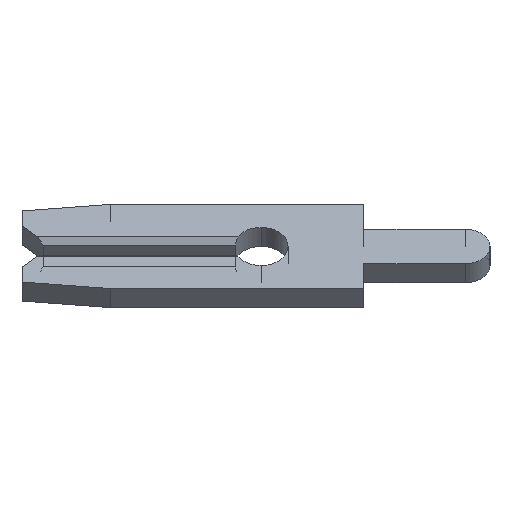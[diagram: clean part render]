
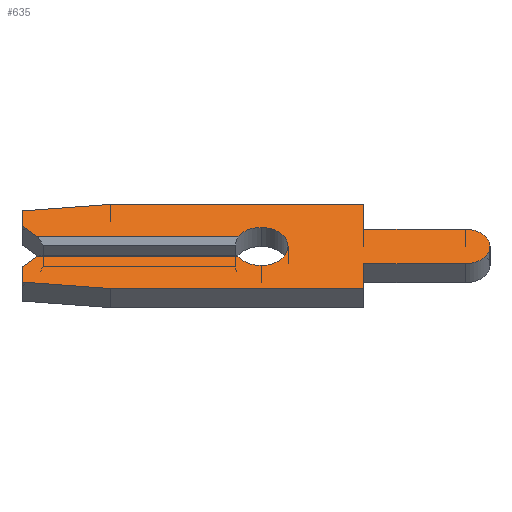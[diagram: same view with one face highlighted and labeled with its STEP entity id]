
A CAD part, left-side view. The second image highlights one B-rep face of the part: STEP entity #635.
In plain terms, the highlighted face is planar.
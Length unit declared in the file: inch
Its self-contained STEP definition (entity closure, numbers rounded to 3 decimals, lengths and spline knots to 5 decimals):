
#38 = EDGE_CURVE ( 'NONE', #1120, #1003, #626, .T. ) ;
#79 = EDGE_CURVE ( 'NONE', #2092, #1792, #140, .T. ) ;
#87 = VERTEX_POINT ( 'NONE', #257 ) ;
#112 = VECTOR ( 'NONE', #1961, 39.37008 ) ;
#115 = VERTEX_POINT ( 'NONE', #1162 ) ;
#116 = CARTESIAN_POINT ( 'NONE',  ( -0.013, -0.099, -0.0575 ) ) ;
#125 = CARTESIAN_POINT ( 'NONE',  ( -0.013, 0.231, 0.04857 ) ) ;
#134 = DIRECTION ( 'NONE',  ( 0., -1., 0. ) ) ;
#140 = CIRCLE ( 'NONE', #2225, 0.026 ) ;
#150 = VERTEX_POINT ( 'NONE', #699 ) ;
#176 = CARTESIAN_POINT ( 'NONE',  ( -0.013, 0.146, -0.0575 ) ) ;
#189 = ORIENTED_EDGE ( 'NONE', *, *, #464, .F. ) ;
#194 = VERTEX_POINT ( 'NONE', #485 ) ;
#195 = EDGE_CURVE ( 'NONE', #227, #2071, #1377, .T. ) ;
#225 = VECTOR ( 'NONE', #446, 39.37008 ) ;
#227 = VERTEX_POINT ( 'NONE', #308 ) ;
#232 = ORIENTED_EDGE ( 'NONE', *, *, #1086, .F. ) ;
#257 = CARTESIAN_POINT ( 'NONE',  ( -0.013, 0.231, 0.028 ) ) ;
#308 = CARTESIAN_POINT ( 'NONE',  ( -0.013, 0.231, 0.04857 ) ) ;
#312 = VECTOR ( 'NONE', #756, 39.37008 ) ;
#326 = EDGE_CURVE ( 'NONE', #115, #2092, #964, .T. ) ;
#348 = DIRECTION ( 'NONE',  ( 0., 0.707, 0.707 ) ) ;
#369 = DIRECTION ( 'NONE',  ( 0., 0.995, 0.105 ) ) ;
#387 = CARTESIAN_POINT ( 'NONE',  ( -0.013, -0.099, -0.0235 ) ) ;
#400 = CARTESIAN_POINT ( 'NONE',  ( -0.013, -0.1975, -0.0235 ) ) ;
#416 = DIRECTION ( 'NONE',  ( 0., 0., 1. ) ) ;
#424 = VECTOR ( 'NONE', #671, 39.37008 ) ;
#426 = CARTESIAN_POINT ( 'NONE',  ( -0.013, 0., 0. ) ) ;
#443 = CARTESIAN_POINT ( 'NONE',  ( -0.013, -0.099, -0.0235 ) ) ;
#446 = DIRECTION ( 'NONE',  ( 0., -1., 0. ) ) ;
#450 = EDGE_CURVE ( 'NONE', #1792, #150, #1846, .T. ) ;
#464 = EDGE_CURVE ( 'NONE', #150, #2282, #1625, .T. ) ;
#485 = CARTESIAN_POINT ( 'NONE',  ( -0.013, -0.099, 0.0575 ) ) ;
#487 = ORIENTED_EDGE ( 'NONE', *, *, #1054, .F. ) ;
#493 = EDGE_CURVE ( 'NONE', #87, #227, #1459, .T. ) ;
#513 = VECTOR ( 'NONE', #134, 39.37008 ) ;
#520 = ORIENTED_EDGE ( 'NONE', *, *, #450, .F. ) ;
#523 = DIRECTION ( 'NONE',  ( -1., 0., 0. ) ) ;
#560 = AXIS2_PLACEMENT_3D ( 'NONE', #2026, #946, #416 ) ;
#565 = LINE ( 'NONE', #848, #1104 ) ;
#591 = LINE ( 'NONE', #1221, #1989 ) ;
#601 = VERTEX_POINT ( 'NONE', #2160 ) ;
#602 = EDGE_CURVE ( 'NONE', #1603, #87, #1551, .T. ) ;
#626 = LINE ( 'NONE', #1579, #225 ) ;
#634 = DIRECTION ( 'NONE',  ( 0., -0.707, 0.707 ) ) ;
#635 = ADVANCED_FACE ( 'NONE', ( #906 ), #730, .F. ) ;
#647 = EDGE_CURVE ( 'NONE', #1382, #921, #1400, .T. ) ;
#671 = DIRECTION ( 'NONE',  ( 0., -0.995, 0.105 ) ) ;
#684 = DIRECTION ( 'NONE',  ( 0., 0., -1. ) ) ;
#686 = ORIENTED_EDGE ( 'NONE', *, *, #326, .F. ) ;
#690 = ORIENTED_EDGE ( 'NONE', *, *, #701, .F. ) ;
#699 = CARTESIAN_POINT ( 'NONE',  ( -0.013, 0., 0.026 ) ) ;
#701 = EDGE_CURVE ( 'NONE', #921, #601, #2284, .T. ) ;
#705 = VECTOR ( 'NONE', #634, 39.37008 ) ;
#729 = LINE ( 'NONE', #116, #1910 ) ;
#730 = PLANE ( 'NONE',  #1295 ) ;
#734 = ORIENTED_EDGE ( 'NONE', *, *, #1749, .F. ) ;
#738 = ORIENTED_EDGE ( 'NONE', *, *, #2148, .F. ) ;
#756 = DIRECTION ( 'NONE',  ( 0., 0., 1. ) ) ;
#786 = LINE ( 'NONE', #1552, #705 ) ;
#816 = ORIENTED_EDGE ( 'NONE', *, *, #647, .F. ) ;
#848 = CARTESIAN_POINT ( 'NONE',  ( -0.013, -0.099, 0.0575 ) ) ;
#876 = DIRECTION ( 'NONE',  ( 0., -1., 0. ) ) ;
#879 = ORIENTED_EDGE ( 'NONE', *, *, #493, .F. ) ;
#880 = VECTOR ( 'NONE', #348, 39.37008 ) ;
#893 = DIRECTION ( 'NONE',  ( 0., 1., 0. ) ) ;
#906 = FACE_OUTER_BOUND ( 'NONE', #2083, .T. ) ;
#907 = CARTESIAN_POINT ( 'NONE',  ( -0.013, 0., 0. ) ) ;
#921 = VERTEX_POINT ( 'NONE', #2195 ) ;
#936 = CARTESIAN_POINT ( 'NONE',  ( -0.013, 0.231, -0.028 ) ) ;
#946 = DIRECTION ( 'NONE',  ( 1., 0., 0. ) ) ;
#963 = CARTESIAN_POINT ( 'NONE',  ( -0.013, -0.099, -0.0575 ) ) ;
#964 = LINE ( 'NONE', #1526, #513 ) ;
#998 = VECTOR ( 'NONE', #369, 39.37008 ) ;
#1001 = AXIS2_PLACEMENT_3D ( 'NONE', #1237, #523, #1784 ) ;
#1003 = VERTEX_POINT ( 'NONE', #2171 ) ;
#1017 = EDGE_CURVE ( 'NONE', #1003, #1312, #2193, .T. ) ;
#1032 = DIRECTION ( 'NONE',  ( 0., 0., -1. ) ) ;
#1039 = CARTESIAN_POINT ( 'NONE',  ( -0.013, 0.231, 0.013 ) ) ;
#1046 = AXIS2_PLACEMENT_3D ( 'NONE', #2166, #1954, #684 ) ;
#1051 = CARTESIAN_POINT ( 'NONE',  ( -0.013, 0.231, 0.028 ) ) ;
#1052 = ORIENTED_EDGE ( 'NONE', *, *, #2218, .F. ) ;
#1054 = EDGE_CURVE ( 'NONE', #1312, #1431, #2306, .T. ) ;
#1086 = EDGE_CURVE ( 'NONE', #601, #1203, #1816, .T. ) ;
#1104 = VECTOR ( 'NONE', #2132, 39.37008 ) ;
#1120 = VERTEX_POINT ( 'NONE', #1131 ) ;
#1131 = CARTESIAN_POINT ( 'NONE',  ( -0.013, -0.099, 0.0235 ) ) ;
#1162 = CARTESIAN_POINT ( 'NONE',  ( -0.013, 0.216, -0.013 ) ) ;
#1177 = ORIENTED_EDGE ( 'NONE', *, *, #1017, .F. ) ;
#1183 = ORIENTED_EDGE ( 'NONE', *, *, #195, .F. ) ;
#1203 = VERTEX_POINT ( 'NONE', #2032 ) ;
#1221 = CARTESIAN_POINT ( 'NONE',  ( -0.013, 0.146, 0.0575 ) ) ;
#1225 = DIRECTION ( 'NONE',  ( 0., -1., 0. ) ) ;
#1234 = CARTESIAN_POINT ( 'NONE',  ( -0.013, 0.02252, -0.013 ) ) ;
#1237 = CARTESIAN_POINT ( 'NONE',  ( -0.013, 0., 0. ) ) ;
#1264 = ORIENTED_EDGE ( 'NONE', *, *, #38, .F. ) ;
#1267 = CARTESIAN_POINT ( 'NONE',  ( -0.013, 0.02252, 0.013 ) ) ;
#1295 = AXIS2_PLACEMENT_3D ( 'NONE', #907, #2002, #2182 ) ;
#1312 = VERTEX_POINT ( 'NONE', #400 ) ;
#1324 = ORIENTED_EDGE ( 'NONE', *, *, #602, .F. ) ;
#1359 = DIRECTION ( 'NONE',  ( -1., 0., 0. ) ) ;
#1377 = LINE ( 'NONE', #125, #424 ) ;
#1382 = VERTEX_POINT ( 'NONE', #963 ) ;
#1400 = LINE ( 'NONE', #176, #2227 ) ;
#1431 = VERTEX_POINT ( 'NONE', #443 ) ;
#1459 = LINE ( 'NONE', #1051, #112 ) ;
#1471 = CARTESIAN_POINT ( 'NONE',  ( -0.013, 0.231, -0.04857 ) ) ;
#1515 = VECTOR ( 'NONE', #1225, 39.37008 ) ;
#1517 = ORIENTED_EDGE ( 'NONE', *, *, #2161, .T. ) ;
#1526 = CARTESIAN_POINT ( 'NONE',  ( -0.013, 0., -0.013 ) ) ;
#1547 = LINE ( 'NONE', #1039, #1515 ) ;
#1551 = LINE ( 'NONE', #1588, #880 ) ;
#1552 = CARTESIAN_POINT ( 'NONE',  ( -0.013, 0.2105, -0.0075 ) ) ;
#1579 = CARTESIAN_POINT ( 'NONE',  ( -0.013, -0.099, 0.0235 ) ) ;
#1588 = CARTESIAN_POINT ( 'NONE',  ( -0.013, 0.2105, 0.0075 ) ) ;
#1603 = VERTEX_POINT ( 'NONE', #1720 ) ;
#1625 = CIRCLE ( 'NONE', #1001, 0.026 ) ;
#1720 = CARTESIAN_POINT ( 'NONE',  ( -0.013, 0.216, 0.013 ) ) ;
#1741 = VECTOR ( 'NONE', #893, 39.37008 ) ;
#1749 = EDGE_CURVE ( 'NONE', #1203, #115, #786, .T. ) ;
#1750 = CARTESIAN_POINT ( 'NONE',  ( -0.013, 0.146, 0.0575 ) ) ;
#1784 = DIRECTION ( 'NONE',  ( 0., 0., -1. ) ) ;
#1792 = VERTEX_POINT ( 'NONE', #1911 ) ;
#1808 = DIRECTION ( 'NONE',  ( 0., 1., 0. ) ) ;
#1816 = LINE ( 'NONE', #936, #312 ) ;
#1846 = CIRCLE ( 'NONE', #1046, 0.026 ) ;
#1875 = ORIENTED_EDGE ( 'NONE', *, *, #2035, .F. ) ;
#1910 = VECTOR ( 'NONE', #2116, 39.37008 ) ;
#1911 = CARTESIAN_POINT ( 'NONE',  ( -0.013, 0., -0.026 ) ) ;
#1920 = ORIENTED_EDGE ( 'NONE', *, *, #79, .F. ) ;
#1954 = DIRECTION ( 'NONE',  ( -1., 0., 0. ) ) ;
#1961 = DIRECTION ( 'NONE',  ( 0., 0., 1. ) ) ;
#1989 = VECTOR ( 'NONE', #876, 39.37008 ) ;
#2002 = DIRECTION ( 'NONE',  ( 1., 0., 0. ) ) ;
#2026 = CARTESIAN_POINT ( 'NONE',  ( -0.013, -0.1975, 0. ) ) ;
#2032 = CARTESIAN_POINT ( 'NONE',  ( -0.013, 0.231, -0.028 ) ) ;
#2035 = EDGE_CURVE ( 'NONE', #1431, #1382, #729, .T. ) ;
#2071 = VERTEX_POINT ( 'NONE', #1750 ) ;
#2083 = EDGE_LOOP ( 'NONE', ( #1517, #189, #520, #1920, #686, #734, #232, #690, #816, #1875, #487, #1177, #1264, #738, #1052, #1183, #879, #1324 ) ) ;
#2092 = VERTEX_POINT ( 'NONE', #1234 ) ;
#2116 = DIRECTION ( 'NONE',  ( 0., 0., -1. ) ) ;
#2132 = DIRECTION ( 'NONE',  ( 0., 0., -1. ) ) ;
#2148 = EDGE_CURVE ( 'NONE', #194, #1120, #565, .T. ) ;
#2160 = CARTESIAN_POINT ( 'NONE',  ( -0.013, 0.231, -0.04857 ) ) ;
#2161 = EDGE_CURVE ( 'NONE', #1603, #2282, #1547, .T. ) ;
#2166 = CARTESIAN_POINT ( 'NONE',  ( -0.013, 0., 0. ) ) ;
#2171 = CARTESIAN_POINT ( 'NONE',  ( -0.013, -0.1975, 0.0235 ) ) ;
#2182 = DIRECTION ( 'NONE',  ( 0., 0., -1. ) ) ;
#2193 = CIRCLE ( 'NONE', #560, 0.0235 ) ;
#2195 = CARTESIAN_POINT ( 'NONE',  ( -0.013, 0.146, -0.0575 ) ) ;
#2218 = EDGE_CURVE ( 'NONE', #2071, #194, #591, .T. ) ;
#2225 = AXIS2_PLACEMENT_3D ( 'NONE', #426, #1359, #1032 ) ;
#2227 = VECTOR ( 'NONE', #1808, 39.37008 ) ;
#2282 = VERTEX_POINT ( 'NONE', #1267 ) ;
#2284 = LINE ( 'NONE', #1471, #998 ) ;
#2306 = LINE ( 'NONE', #387, #1741 ) ;
